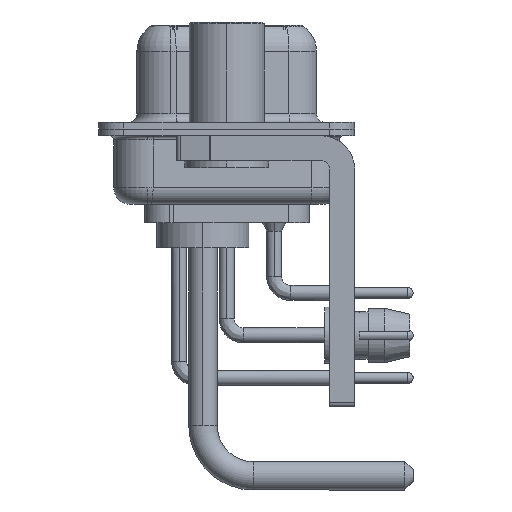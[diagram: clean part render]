
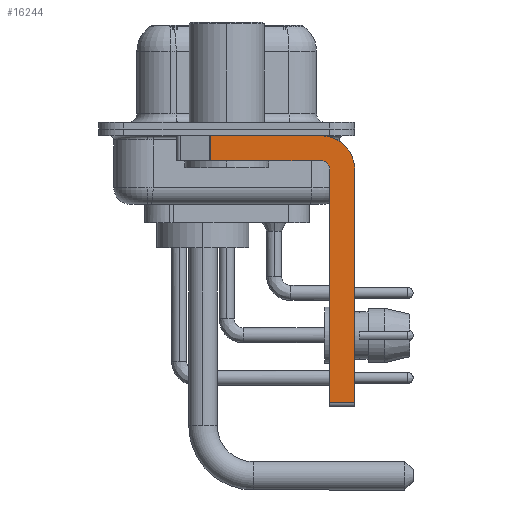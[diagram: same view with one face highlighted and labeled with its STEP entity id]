
A CAD part, left-side view. The second image highlights one B-rep face of the part: STEP entity #16244.
In plain terms, the highlighted planar face has unit normal (-1, 0, 0).
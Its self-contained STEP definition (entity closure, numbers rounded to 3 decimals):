
#51 = EDGE_CURVE ( 'NONE', #19618, #19732, #9980, .T. ) ;
#265 = VECTOR ( 'NONE', #17000, 1000. ) ;
#1048 = DIRECTION ( 'NONE',  ( 0., 0., -1. ) ) ;
#1147 = CARTESIAN_POINT ( 'NONE',  ( -2.9, -6.15, -16.6 ) ) ;
#1202 = VERTEX_POINT ( 'NONE', #28793 ) ;
#2108 = VECTOR ( 'NONE', #20112, 1000. ) ;
#2328 = PLANE ( 'NONE',  #20811 ) ;
#3830 = VECTOR ( 'NONE', #6101, 1000. ) ;
#3876 = ORIENTED_EDGE ( 'NONE', *, *, #30262, .F. ) ;
#4379 = VECTOR ( 'NONE', #24047, 1000. ) ;
#4424 = CIRCLE ( 'NONE', #10250, 2. ) ;
#4763 = VERTEX_POINT ( 'NONE', #22190 ) ;
#4841 = DIRECTION ( 'NONE',  ( 0., 0., -1. ) ) ;
#5162 = EDGE_LOOP ( 'NONE', ( #3876, #23417, #21977, #8131, #25752, #12942, #29111, #6298 ) ) ;
#5314 = CARTESIAN_POINT ( 'NONE',  ( -2.9, 0.978, -1.9 ) ) ;
#5996 = LINE ( 'NONE', #1147, #28820 ) ;
#6101 = DIRECTION ( 'NONE',  ( 0., -1., 0. ) ) ;
#6229 = CARTESIAN_POINT ( 'NONE',  ( -2.9, -7.65, -2.4 ) ) ;
#6298 = ORIENTED_EDGE ( 'NONE', *, *, #32349, .F. ) ;
#6322 = DIRECTION ( 'NONE',  ( -1., 0., 0. ) ) ;
#6593 = LINE ( 'NONE', #26688, #4379 ) ;
#6872 = CARTESIAN_POINT ( 'NONE',  ( -2.9, -5.65, -16.35 ) ) ;
#6881 = CARTESIAN_POINT ( 'NONE',  ( -2.9, -5.65, -2.4 ) ) ;
#8131 = ORIENTED_EDGE ( 'NONE', *, *, #24107, .F. ) ;
#8322 = CARTESIAN_POINT ( 'NONE',  ( -2.9, -6.15, -2.4 ) ) ;
#8727 = DIRECTION ( 'NONE',  ( 1., 0., 0. ) ) ;
#9075 = CARTESIAN_POINT ( 'NONE',  ( -2.9, 0.978, -1.9 ) ) ;
#9980 = LINE ( 'NONE', #5314, #2108 ) ;
#10250 = AXIS2_PLACEMENT_3D ( 'NONE', #6881, #8727, #11363 ) ;
#11363 = DIRECTION ( 'NONE',  ( 0., 0., -1. ) ) ;
#12942 = ORIENTED_EDGE ( 'NONE', *, *, #20247, .T. ) ;
#13642 = VERTEX_POINT ( 'NONE', #8322 ) ;
#14799 = CARTESIAN_POINT ( 'NONE',  ( -2.9, -5.65, -2.4 ) ) ;
#16244 = ADVANCED_FACE ( 'NONE', ( #32611 ), #2328, .F. ) ;
#16287 = DIRECTION ( 'NONE',  ( 0., 0., 1. ) ) ;
#16462 = EDGE_CURVE ( 'NONE', #24844, #13642, #5996, .T. ) ;
#17000 = DIRECTION ( 'NONE',  ( 0., -1., 0. ) ) ;
#17637 = DIRECTION ( 'NONE',  ( 1., 0., 0. ) ) ;
#18437 = CIRCLE ( 'NONE', #26373, 0.5 ) ;
#18563 = CARTESIAN_POINT ( 'NONE',  ( -2.9, 3., -0.4 ) ) ;
#19618 = VERTEX_POINT ( 'NONE', #25539 ) ;
#19732 = VERTEX_POINT ( 'NONE', #9075 ) ;
#20112 = DIRECTION ( 'NONE',  ( 0., 0., -1. ) ) ;
#20247 = EDGE_CURVE ( 'NONE', #24844, #4763, #27308, .T. ) ;
#20346 = VECTOR ( 'NONE', #1048, 1000. ) ;
#20811 = AXIS2_PLACEMENT_3D ( 'NONE', #14799, #17637, #4841 ) ;
#21057 = LINE ( 'NONE', #18563, #3830 ) ;
#21683 = CARTESIAN_POINT ( 'NONE',  ( -2.9, -6.15, -16.35 ) ) ;
#21977 = ORIENTED_EDGE ( 'NONE', *, *, #30379, .F. ) ;
#22190 = CARTESIAN_POINT ( 'NONE',  ( -2.9, -7.65, -16.35 ) ) ;
#22749 = CARTESIAN_POINT ( 'NONE',  ( -2.9, -7.65, -2.4 ) ) ;
#22993 = CARTESIAN_POINT ( 'NONE',  ( -2.9, -5.65, -0.4 ) ) ;
#23417 = ORIENTED_EDGE ( 'NONE', *, *, #51, .T. ) ;
#23542 = VERTEX_POINT ( 'NONE', #22993 ) ;
#24047 = DIRECTION ( 'NONE',  ( 0., 1., 0. ) ) ;
#24107 = EDGE_CURVE ( 'NONE', #13642, #1202, #18437, .T. ) ;
#24844 = VERTEX_POINT ( 'NONE', #21683 ) ;
#25539 = CARTESIAN_POINT ( 'NONE',  ( -2.9, 0.978, -0.4 ) ) ;
#25752 = ORIENTED_EDGE ( 'NONE', *, *, #16462, .F. ) ;
#26373 = AXIS2_PLACEMENT_3D ( 'NONE', #29095, #6322, #16287 ) ;
#26688 = CARTESIAN_POINT ( 'NONE',  ( -2.9, -5.65, -1.9 ) ) ;
#27273 = VERTEX_POINT ( 'NONE', #22749 ) ;
#27308 = LINE ( 'NONE', #6872, #265 ) ;
#28793 = CARTESIAN_POINT ( 'NONE',  ( -2.9, -5.65, -1.9 ) ) ;
#28820 = VECTOR ( 'NONE', #31416, 1000. ) ;
#29095 = CARTESIAN_POINT ( 'NONE',  ( -2.9, -5.65, -2.4 ) ) ;
#29111 = ORIENTED_EDGE ( 'NONE', *, *, #32343, .F. ) ;
#29158 = LINE ( 'NONE', #6229, #20346 ) ;
#30262 = EDGE_CURVE ( 'NONE', #19618, #23542, #21057, .T. ) ;
#30379 = EDGE_CURVE ( 'NONE', #1202, #19732, #6593, .T. ) ;
#31416 = DIRECTION ( 'NONE',  ( 0., 0., 1. ) ) ;
#32343 = EDGE_CURVE ( 'NONE', #27273, #4763, #29158, .T. ) ;
#32349 = EDGE_CURVE ( 'NONE', #23542, #27273, #4424, .T. ) ;
#32611 = FACE_OUTER_BOUND ( 'NONE', #5162, .T. ) ;
